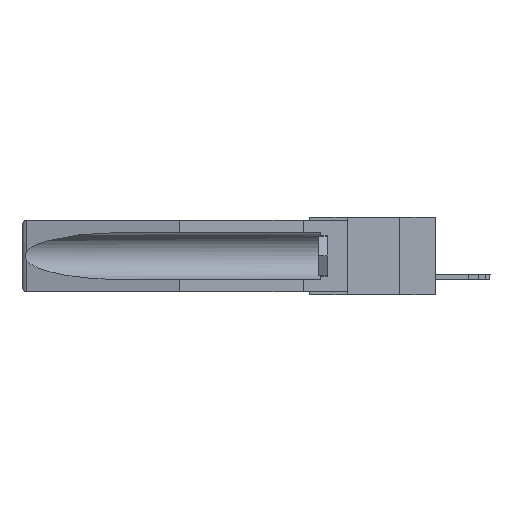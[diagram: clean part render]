
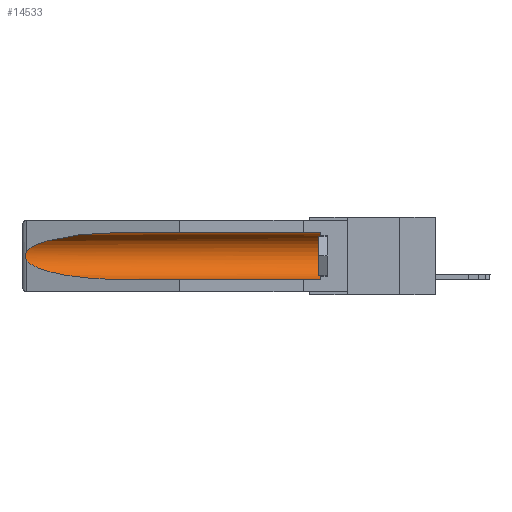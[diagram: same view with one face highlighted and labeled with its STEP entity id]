
A CAD part, left-side view. The second image highlights one B-rep face of the part: STEP entity #14533.
In plain terms, the highlighted cylindrical face has radius 2.857 mm (diameter 5.715 mm), a partial arc.
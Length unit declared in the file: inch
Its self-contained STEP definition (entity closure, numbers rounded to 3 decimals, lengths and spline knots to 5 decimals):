
#362 = CARTESIAN_POINT ( 'NONE',  ( 0.26597, 1.5296, -0.19026 ) ) ;
#515 = B_SPLINE_CURVE_WITH_KNOTS ( 'NONE', 3,
 ( #3084, #8234, #7009, #16156, #16261, #4256, #16317, #14938, #362, #9650 ),
 .UNSPECIFIED., .F., .F.,
 ( 4, 2, 2, 2, 4 ),
 ( 0., 0.00029, 0.00058, 0.00087, 0.00117 ),
 .UNSPECIFIED. ) ;
#648 = CARTESIAN_POINT ( 'NONE',  ( 0.21114, 1.30732, -0.284 ) ) ;
#816 = CARTESIAN_POINT ( 'NONE',  ( 0.155, -0.30754, -0.284 ) ) ;
#1225 = CARTESIAN_POINT ( 'NONE',  ( 0.26537, 1.52718, -0.14972 ) ) ;
#1604 = VECTOR ( 'NONE', #10099, 39.37008 ) ;
#2157 = DIRECTION ( 'NONE',  ( 0., 0., 1. ) ) ;
#2342 = EDGE_CURVE ( 'NONE', #15628, #6656, #515, .T. ) ;
#2402 = EDGE_CURVE ( 'NONE', #6656, #15494, #15127, .T. ) ;
#3084 = CARTESIAN_POINT ( 'NONE',  ( 0.26537, 1.52718, -0.14972 ) ) ;
#3127 = VECTOR ( 'NONE', #3434, 39.37008 ) ;
#3179 = EDGE_CURVE ( 'NONE', #11814, #15628, #5425, .T. ) ;
#3434 = DIRECTION ( 'NONE',  ( 0., 1., 0. ) ) ;
#3686 = LINE ( 'NONE', #11074, #1604 ) ;
#4256 = CARTESIAN_POINT ( 'NONE',  ( 0.2675, 1.53308, -0.17534 ) ) ;
#4278 = CARTESIAN_POINT ( 'NONE',  ( 0.155, 0.126, -0.284 ) ) ;
#4285 = DIRECTION ( 'NONE',  ( 0., 1., 0. ) ) ;
#4570 = CARTESIAN_POINT ( 'NONE',  ( 0.155, 1.07973, -0.059 ) ) ;
#5236 = ORIENTED_EDGE ( 'NONE', *, *, #2402, .T. ) ;
#5425 =( BOUNDED_CURVE ( )  B_SPLINE_CURVE ( 3, ( #4570, #7198, #13628, #8427 ),
 .UNSPECIFIED., .F., .F. ) 
 B_SPLINE_CURVE_WITH_KNOTS ( ( 4, 4 ),
 ( 4.71239, 6.08839 ),
 .UNSPECIFIED. ) 
 CURVE ( )  GEOMETRIC_REPRESENTATION_ITEM ( )  RATIONAL_B_SPLINE_CURVE ( ( 1., 0.848, 0.848, 1. ) ) 
 REPRESENTATION_ITEM ( '' )  );
#5831 = CARTESIAN_POINT ( 'NONE',  ( 0.25451, 1.48313, -0.24835 ) ) ;
#6173 = CARTESIAN_POINT ( 'NONE',  ( 0.155, -0.30754, -0.1715 ) ) ;
#6356 = CARTESIAN_POINT ( 'NONE',  ( 0.155, 0.126, -0.059 ) ) ;
#6656 = VERTEX_POINT ( 'NONE', #16492 ) ;
#7009 = CARTESIAN_POINT ( 'NONE',  ( 0.26654, 1.53092, -0.15636 ) ) ;
#7198 = CARTESIAN_POINT ( 'NONE',  ( 0.21114, 1.30732, -0.059 ) ) ;
#7777 = VERTEX_POINT ( 'NONE', #4278 ) ;
#8234 = CARTESIAN_POINT ( 'NONE',  ( 0.26597, 1.52961, -0.15275 ) ) ;
#8427 = CARTESIAN_POINT ( 'NONE',  ( 0.26537, 1.52718, -0.14972 ) ) ;
#8511 = FACE_OUTER_BOUND ( 'NONE', #12682, .T. ) ;
#9618 = ORIENTED_EDGE ( 'NONE', *, *, #3179, .T. ) ;
#9634 = AXIS2_PLACEMENT_3D ( 'NONE', #6173, #4285, #16070 ) ;
#9650 = CARTESIAN_POINT ( 'NONE',  ( 0.26537, 1.52718, -0.19328 ) ) ;
#9930 = CARTESIAN_POINT ( 'NONE',  ( 0.155, 1.07973, -0.284 ) ) ;
#9932 = DIRECTION ( 'NONE',  ( 0., -1., 0. ) ) ;
#10023 = CIRCLE ( 'NONE', #16234, 0.1125 ) ;
#10099 = DIRECTION ( 'NONE',  ( 0., 1., 0. ) ) ;
#10269 = ORIENTED_EDGE ( 'NONE', *, *, #16245, .T. ) ;
#10370 = ORIENTED_EDGE ( 'NONE', *, *, #2342, .T. ) ;
#11074 = CARTESIAN_POINT ( 'NONE',  ( 0.155, -0.30754, -0.059 ) ) ;
#11200 = CARTESIAN_POINT ( 'NONE',  ( 0.155, 0.126, -0.1715 ) ) ;
#11814 = VERTEX_POINT ( 'NONE', #13264 ) ;
#12016 = ORIENTED_EDGE ( 'NONE', *, *, #13884, .F. ) ;
#12080 = EDGE_CURVE ( 'NONE', #7777, #12194, #10023, .T. ) ;
#12194 = VERTEX_POINT ( 'NONE', #6356 ) ;
#12535 = CARTESIAN_POINT ( 'NONE',  ( 0.155, 1.07973, -0.284 ) ) ;
#12682 = EDGE_LOOP ( 'NONE', ( #9618, #10370, #5236, #12016, #15835, #10269 ) ) ;
#13264 = CARTESIAN_POINT ( 'NONE',  ( 0.155, 1.07973, -0.059 ) ) ;
#13628 = CARTESIAN_POINT ( 'NONE',  ( 0.25451, 1.48313, -0.09465 ) ) ;
#13823 = CARTESIAN_POINT ( 'NONE',  ( 0.26537, 1.52718, -0.19328 ) ) ;
#13884 = EDGE_CURVE ( 'NONE', #7777, #15494, #17003, .T. ) ;
#14533 = ADVANCED_FACE ( 'NONE', ( #8511 ), #16534, .F. ) ;
#14938 = CARTESIAN_POINT ( 'NONE',  ( 0.26655, 1.53094, -0.18657 ) ) ;
#15127 =( BOUNDED_CURVE ( )  B_SPLINE_CURVE ( 3, ( #13823, #5831, #648, #9930 ),
 .UNSPECIFIED., .F., .T. ) 
 B_SPLINE_CURVE_WITH_KNOTS ( ( 4, 4 ),
 ( 0.1948, 1.5708 ),
 .UNSPECIFIED. ) 
 CURVE ( )  GEOMETRIC_REPRESENTATION_ITEM ( )  RATIONAL_B_SPLINE_CURVE ( ( 1., 0.848, 0.848, 1. ) ) 
 REPRESENTATION_ITEM ( '' )  );
#15494 = VERTEX_POINT ( 'NONE', #12535 ) ;
#15628 = VERTEX_POINT ( 'NONE', #1225 ) ;
#15835 = ORIENTED_EDGE ( 'NONE', *, *, #12080, .T. ) ;
#16070 = DIRECTION ( 'NONE',  ( 0., 0., 1. ) ) ;
#16156 = CARTESIAN_POINT ( 'NONE',  ( 0.2673, 1.5327, -0.16383 ) ) ;
#16234 = AXIS2_PLACEMENT_3D ( 'NONE', #11200, #9932, #2157 ) ;
#16245 = EDGE_CURVE ( 'NONE', #12194, #11814, #3686, .T. ) ;
#16261 = CARTESIAN_POINT ( 'NONE',  ( 0.2675, 1.53308, -0.16763 ) ) ;
#16317 = CARTESIAN_POINT ( 'NONE',  ( 0.2673, 1.53269, -0.17917 ) ) ;
#16492 = CARTESIAN_POINT ( 'NONE',  ( 0.26537, 1.52718, -0.19328 ) ) ;
#16534 = CYLINDRICAL_SURFACE ( 'NONE', #9634, 0.1125 ) ;
#17003 = LINE ( 'NONE', #816, #3127 ) ;
